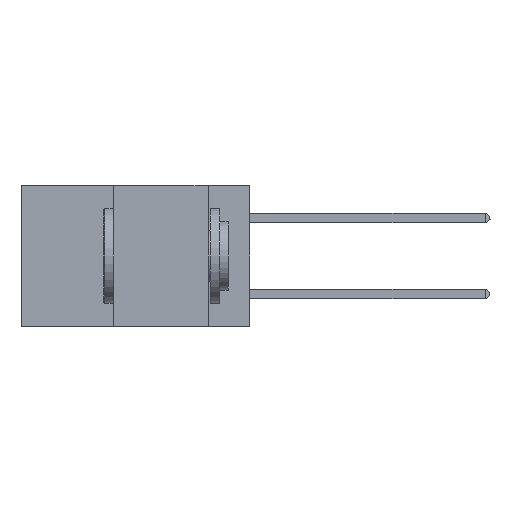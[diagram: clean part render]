
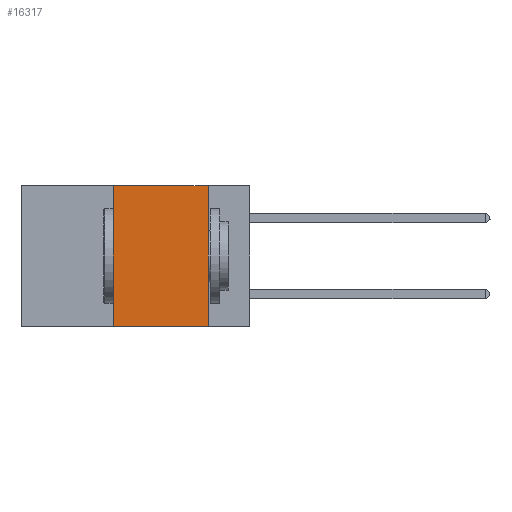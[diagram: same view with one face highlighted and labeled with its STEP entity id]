
A CAD part, left-side view. The second image highlights one B-rep face of the part: STEP entity #16317.
In plain terms, the highlighted planar face has unit normal (-1, 0, 0).
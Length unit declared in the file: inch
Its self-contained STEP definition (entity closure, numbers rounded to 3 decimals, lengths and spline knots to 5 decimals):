
#406 = DIRECTION ( 'NONE',  ( 1., 0., 0. ) ) ;
#569 = VERTEX_POINT ( 'NONE', #14943 ) ;
#1084 = DIRECTION ( 'NONE',  ( 0., -1., 0. ) ) ;
#1149 = LINE ( 'NONE', #9784, #4908 ) ;
#1272 = EDGE_CURVE ( 'NONE', #14871, #569, #5270, .T. ) ;
#1648 = VECTOR ( 'NONE', #11257, 39.37008 ) ;
#2157 = LINE ( 'NONE', #12792, #1648 ) ;
#2896 = LINE ( 'NONE', #4398, #10664 ) ;
#3553 = FACE_OUTER_BOUND ( 'NONE', #6239, .T. ) ;
#4398 = CARTESIAN_POINT ( 'NONE',  ( 0., 0.6, 0. ) ) ;
#4410 = CARTESIAN_POINT ( 'NONE',  ( 0., 0.36, 0. ) ) ;
#4908 = VECTOR ( 'NONE', #5194, 39.37008 ) ;
#4920 = ORIENTED_EDGE ( 'NONE', *, *, #18322, .F. ) ;
#5194 = DIRECTION ( 'NONE',  ( 0., 0., -1. ) ) ;
#5270 = LINE ( 'NONE', #12829, #16564 ) ;
#5366 = ORIENTED_EDGE ( 'NONE', *, *, #20011, .F. ) ;
#5574 = ORIENTED_EDGE ( 'NONE', *, *, #18289, .F. ) ;
#6239 = EDGE_LOOP ( 'NONE', ( #4920, #5366, #5574, #6685 ) ) ;
#6685 = ORIENTED_EDGE ( 'NONE', *, *, #1272, .T. ) ;
#7785 = VERTEX_POINT ( 'NONE', #4410 ) ;
#8319 = CARTESIAN_POINT ( 'NONE',  ( 0., 0.6, 0. ) ) ;
#8963 = VERTEX_POINT ( 'NONE', #17886 ) ;
#9784 = CARTESIAN_POINT ( 'NONE',  ( 0., 0.11, 0. ) ) ;
#10664 = VECTOR ( 'NONE', #1084, 39.37008 ) ;
#11257 = DIRECTION ( 'NONE',  ( 0., 0., 1. ) ) ;
#11400 = DIRECTION ( 'NONE',  ( 0., 0., -1. ) ) ;
#12764 = DIRECTION ( 'NONE',  ( 0., -1., 0. ) ) ;
#12792 = CARTESIAN_POINT ( 'NONE',  ( 0., 0.36, 0. ) ) ;
#12829 = CARTESIAN_POINT ( 'NONE',  ( 0., 0.6, -0.37 ) ) ;
#14871 = VERTEX_POINT ( 'NONE', #17144 ) ;
#14943 = CARTESIAN_POINT ( 'NONE',  ( 0., 0.11, -0.37 ) ) ;
#15862 = AXIS2_PLACEMENT_3D ( 'NONE', #8319, #406, #11400 ) ;
#16317 = ADVANCED_FACE ( 'NONE', ( #3553 ), #19039, .F. ) ;
#16564 = VECTOR ( 'NONE', #12764, 39.37008 ) ;
#17144 = CARTESIAN_POINT ( 'NONE',  ( 0., 0.36, -0.37 ) ) ;
#17886 = CARTESIAN_POINT ( 'NONE',  ( 0., 0.11, 0. ) ) ;
#18289 = EDGE_CURVE ( 'NONE', #14871, #7785, #2157, .T. ) ;
#18322 = EDGE_CURVE ( 'NONE', #8963, #569, #1149, .T. ) ;
#19039 = PLANE ( 'NONE',  #15862 ) ;
#20011 = EDGE_CURVE ( 'NONE', #7785, #8963, #2896, .T. ) ;
